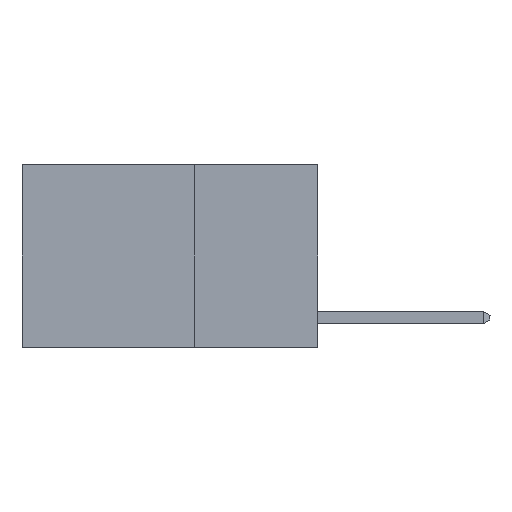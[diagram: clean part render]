
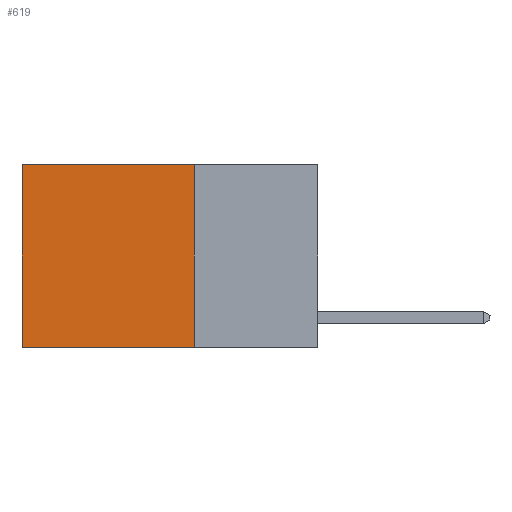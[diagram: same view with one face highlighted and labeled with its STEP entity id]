
A CAD part, left-side view. The second image highlights one B-rep face of the part: STEP entity #619.
In plain terms, the highlighted planar face has unit normal (-1, 0, 0).
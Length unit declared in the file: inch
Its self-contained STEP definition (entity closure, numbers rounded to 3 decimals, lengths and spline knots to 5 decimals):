
#619 = ADVANCED_FACE ( 'NONE', ( #8073 ), #10939, .F. ) ;
#2988 = AXIS2_PLACEMENT_3D ( 'NONE', #11144, #10887, #10823 ) ;
#3245 = CARTESIAN_POINT ( 'NONE',  ( 0.2625, 0.25, -0.37 ) ) ;
#4603 = VERTEX_POINT ( 'NONE', #12296 ) ;
#6443 = EDGE_LOOP ( 'NONE', ( #10480, #19989, #23351, #12330 ) ) ;
#7228 = CARTESIAN_POINT ( 'NONE',  ( 0.2625, 0.25, 0. ) ) ;
#7282 = CARTESIAN_POINT ( 'NONE',  ( 0.2625, 0.25, -0.37 ) ) ;
#7449 = CARTESIAN_POINT ( 'NONE',  ( 0.2625, 0.6, 0. ) ) ;
#8073 = FACE_OUTER_BOUND ( 'NONE', #6443, .T. ) ;
#8195 = VERTEX_POINT ( 'NONE', #7449 ) ;
#8792 = EDGE_CURVE ( 'NONE', #10932, #20027, #15979, .T. ) ;
#9826 = VECTOR ( 'NONE', #21831, 39.37008 ) ;
#10480 = ORIENTED_EDGE ( 'NONE', *, *, #21343, .T. ) ;
#10555 = VECTOR ( 'NONE', #25648, 39.37008 ) ;
#10823 = DIRECTION ( 'NONE',  ( 0., 0., -1. ) ) ;
#10887 = DIRECTION ( 'NONE',  ( 1., 0., 0. ) ) ;
#10932 = VERTEX_POINT ( 'NONE', #26180 ) ;
#10939 = PLANE ( 'NONE',  #2988 ) ;
#11144 = CARTESIAN_POINT ( 'NONE',  ( 0.2625, 0.25, 0. ) ) ;
#12169 = VECTOR ( 'NONE', #13581, 39.37008 ) ;
#12296 = CARTESIAN_POINT ( 'NONE',  ( 0.2625, 0.6, -0.37 ) ) ;
#12330 = ORIENTED_EDGE ( 'NONE', *, *, #23878, .T. ) ;
#12810 = LINE ( 'NONE', #25814, #12169 ) ;
#13581 = DIRECTION ( 'NONE',  ( 0., 0., -1. ) ) ;
#13915 = VECTOR ( 'NONE', #23685, 39.37008 ) ;
#15979 = LINE ( 'NONE', #17361, #10555 ) ;
#17152 = EDGE_CURVE ( 'NONE', #20027, #4603, #20733, .T. ) ;
#17361 = CARTESIAN_POINT ( 'NONE',  ( 0.2625, 0.25, 0. ) ) ;
#19989 = ORIENTED_EDGE ( 'NONE', *, *, #17152, .F. ) ;
#20027 = VERTEX_POINT ( 'NONE', #7282 ) ;
#20733 = LINE ( 'NONE', #3245, #9826 ) ;
#21343 = EDGE_CURVE ( 'NONE', #8195, #4603, #12810, .T. ) ;
#21831 = DIRECTION ( 'NONE',  ( 0., 1., 0. ) ) ;
#23351 = ORIENTED_EDGE ( 'NONE', *, *, #8792, .F. ) ;
#23685 = DIRECTION ( 'NONE',  ( 0., 1., 0. ) ) ;
#23878 = EDGE_CURVE ( 'NONE', #10932, #8195, #24870, .T. ) ;
#24870 = LINE ( 'NONE', #7228, #13915 ) ;
#25648 = DIRECTION ( 'NONE',  ( 0., 0., -1. ) ) ;
#25814 = CARTESIAN_POINT ( 'NONE',  ( 0.2625, 0.6, 0. ) ) ;
#26180 = CARTESIAN_POINT ( 'NONE',  ( 0.2625, 0.25, 0. ) ) ;
